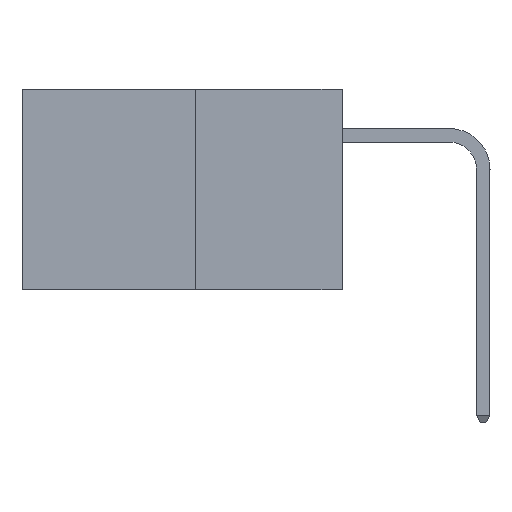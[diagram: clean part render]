
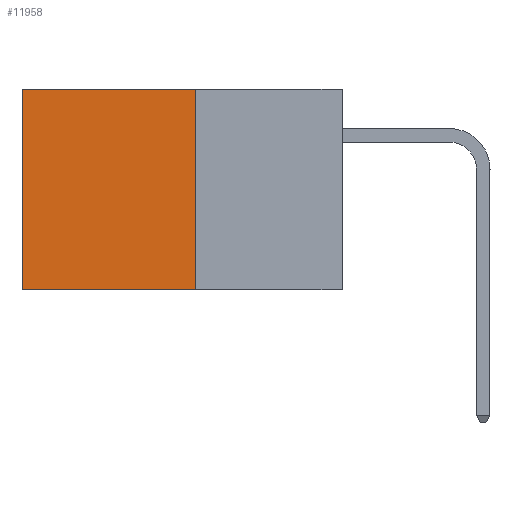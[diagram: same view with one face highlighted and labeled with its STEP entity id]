
A CAD part, left-side view. The second image highlights one B-rep face of the part: STEP entity #11958.
In plain terms, the highlighted planar face has unit normal (-1, 0, 0).
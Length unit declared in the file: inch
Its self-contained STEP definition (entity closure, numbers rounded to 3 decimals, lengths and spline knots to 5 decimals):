
#685 = VECTOR ( 'NONE', #7678, 39.37008 ) ;
#1423 = PLANE ( 'NONE',  #11197 ) ;
#1776 = ORIENTED_EDGE ( 'NONE', *, *, #3651, .F. ) ;
#1912 = CARTESIAN_POINT ( 'NONE',  ( 0.277, 0.27, 0. ) ) ;
#2896 = DIRECTION ( 'NONE',  ( 1., 0., 0. ) ) ;
#3257 = VECTOR ( 'NONE', #14284, 39.37008 ) ;
#3398 = VERTEX_POINT ( 'NONE', #10163 ) ;
#3651 = EDGE_CURVE ( 'NONE', #3398, #5854, #8422, .T. ) ;
#4337 = CARTESIAN_POINT ( 'NONE',  ( 0.277, 0.27, -0.37 ) ) ;
#5072 = VECTOR ( 'NONE', #14711, 39.37008 ) ;
#5771 = DIRECTION ( 'NONE',  ( 0., 1., 0. ) ) ;
#5787 = CARTESIAN_POINT ( 'NONE',  ( 0.277, 0.27, -0.37 ) ) ;
#5854 = VERTEX_POINT ( 'NONE', #8584 ) ;
#6273 = VECTOR ( 'NONE', #5771, 39.37008 ) ;
#7678 = DIRECTION ( 'NONE',  ( 0., 1., 0. ) ) ;
#8045 = VERTEX_POINT ( 'NONE', #8454 ) ;
#8381 = LINE ( 'NONE', #1912, #685 ) ;
#8422 = LINE ( 'NONE', #5787, #3257 ) ;
#8454 = CARTESIAN_POINT ( 'NONE',  ( 0.277, 0.59, -0.37 ) ) ;
#8584 = CARTESIAN_POINT ( 'NONE',  ( 0.277, 0.27, -0.37 ) ) ;
#8757 = ORIENTED_EDGE ( 'NONE', *, *, #17740, .T. ) ;
#9232 = EDGE_LOOP ( 'NONE', ( #8757, #9681, #1776, #9933 ) ) ;
#9681 = ORIENTED_EDGE ( 'NONE', *, *, #9776, .F. ) ;
#9776 = EDGE_CURVE ( 'NONE', #5854, #8045, #10579, .T. ) ;
#9933 = ORIENTED_EDGE ( 'NONE', *, *, #13368, .T. ) ;
#10163 = CARTESIAN_POINT ( 'NONE',  ( 0.277, 0.27, 0. ) ) ;
#10579 = LINE ( 'NONE', #4337, #6273 ) ;
#11197 = AXIS2_PLACEMENT_3D ( 'NONE', #11520, #2896, #12896 ) ;
#11349 = VERTEX_POINT ( 'NONE', #12915 ) ;
#11520 = CARTESIAN_POINT ( 'NONE',  ( 0.277, 0.27, -0.37 ) ) ;
#11958 = ADVANCED_FACE ( 'NONE', ( #16136 ), #1423, .F. ) ;
#12655 = LINE ( 'NONE', #17501, #5072 ) ;
#12896 = DIRECTION ( 'NONE',  ( 0., 0., -1. ) ) ;
#12915 = CARTESIAN_POINT ( 'NONE',  ( 0.277, 0.59, 0. ) ) ;
#13368 = EDGE_CURVE ( 'NONE', #3398, #11349, #8381, .T. ) ;
#14284 = DIRECTION ( 'NONE',  ( 0., 0., -1. ) ) ;
#14711 = DIRECTION ( 'NONE',  ( 0., 0., -1. ) ) ;
#16136 = FACE_OUTER_BOUND ( 'NONE', #9232, .T. ) ;
#17501 = CARTESIAN_POINT ( 'NONE',  ( 0.277, 0.59, -0.37 ) ) ;
#17740 = EDGE_CURVE ( 'NONE', #11349, #8045, #12655, .T. ) ;
